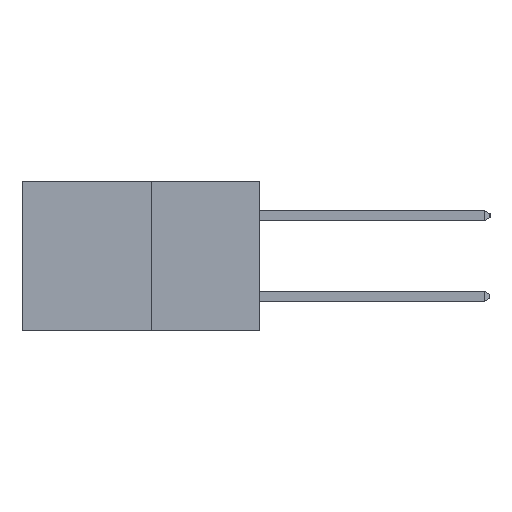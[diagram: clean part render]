
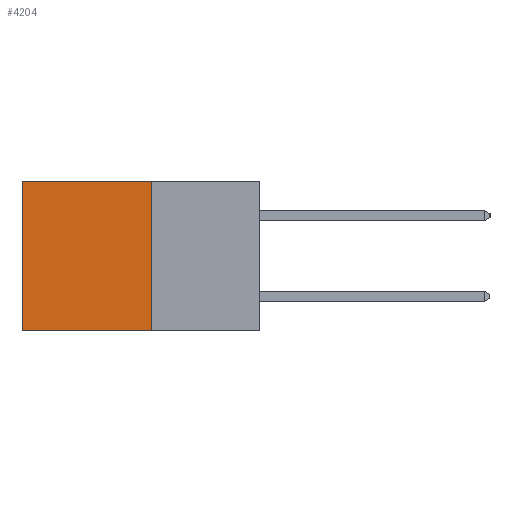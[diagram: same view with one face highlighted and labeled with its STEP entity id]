
A CAD part, left-side view. The second image highlights one B-rep face of the part: STEP entity #4204.
In plain terms, the highlighted planar face has unit normal (-1, 0, 0).
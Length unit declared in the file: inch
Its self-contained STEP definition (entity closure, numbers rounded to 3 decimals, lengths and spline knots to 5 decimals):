
#1042 = AXIS2_PLACEMENT_3D ( 'NONE', #10837, #10666, #10637 ) ;
#1315 = VECTOR ( 'NONE', #5972, 39.37008 ) ;
#1460 = ORIENTED_EDGE ( 'NONE', *, *, #1589, .T. ) ;
#1569 = DIRECTION ( 'NONE',  ( 0., 0., -1. ) ) ;
#1589 = EDGE_CURVE ( 'NONE', #2111, #4474, #9995, .T. ) ;
#1935 = CARTESIAN_POINT ( 'NONE',  ( 0.277, 0.59, -0.37 ) ) ;
#2111 = VERTEX_POINT ( 'NONE', #7039 ) ;
#2406 = CARTESIAN_POINT ( 'NONE',  ( 0.277, 0.27, -0.37 ) ) ;
#2801 = ORIENTED_EDGE ( 'NONE', *, *, #9775, .F. ) ;
#3707 = EDGE_CURVE ( 'NONE', #13446, #10469, #14381, .T. ) ;
#4204 = ADVANCED_FACE ( 'NONE', ( #5277 ), #10990, .F. ) ;
#4474 = VERTEX_POINT ( 'NONE', #10287 ) ;
#4891 = CARTESIAN_POINT ( 'NONE',  ( 0.277, 0.27, -0.37 ) ) ;
#5277 = FACE_OUTER_BOUND ( 'NONE', #15206, .T. ) ;
#5972 = DIRECTION ( 'NONE',  ( 0., 1., 0. ) ) ;
#6163 = CARTESIAN_POINT ( 'NONE',  ( 0.277, 0.27, 0. ) ) ;
#6466 = EDGE_CURVE ( 'NONE', #4474, #10469, #8053, .T. ) ;
#7039 = CARTESIAN_POINT ( 'NONE',  ( 0.277, 0.27, 0. ) ) ;
#7177 = CARTESIAN_POINT ( 'NONE',  ( 0.277, 0.27, -0.37 ) ) ;
#7349 = DIRECTION ( 'NONE',  ( 0., 0., -1. ) ) ;
#7760 = ORIENTED_EDGE ( 'NONE', *, *, #6466, .T. ) ;
#8053 = LINE ( 'NONE', #1935, #10569 ) ;
#8323 = DIRECTION ( 'NONE',  ( 0., 1., 0. ) ) ;
#9321 = LINE ( 'NONE', #4891, #15204 ) ;
#9775 = EDGE_CURVE ( 'NONE', #2111, #13446, #9321, .T. ) ;
#9995 = LINE ( 'NONE', #6163, #1315 ) ;
#10287 = CARTESIAN_POINT ( 'NONE',  ( 0.277, 0.59, 0. ) ) ;
#10469 = VERTEX_POINT ( 'NONE', #11148 ) ;
#10569 = VECTOR ( 'NONE', #1569, 39.37008 ) ;
#10637 = DIRECTION ( 'NONE',  ( 0., 0., -1. ) ) ;
#10666 = DIRECTION ( 'NONE',  ( 1., 0., 0. ) ) ;
#10837 = CARTESIAN_POINT ( 'NONE',  ( 0.277, 0.27, -0.37 ) ) ;
#10886 = VECTOR ( 'NONE', #8323, 39.37008 ) ;
#10990 = PLANE ( 'NONE',  #1042 ) ;
#11148 = CARTESIAN_POINT ( 'NONE',  ( 0.277, 0.59, -0.37 ) ) ;
#11801 = ORIENTED_EDGE ( 'NONE', *, *, #3707, .F. ) ;
#13446 = VERTEX_POINT ( 'NONE', #7177 ) ;
#14381 = LINE ( 'NONE', #2406, #10886 ) ;
#15204 = VECTOR ( 'NONE', #7349, 39.37008 ) ;
#15206 = EDGE_LOOP ( 'NONE', ( #7760, #11801, #2801, #1460 ) ) ;
